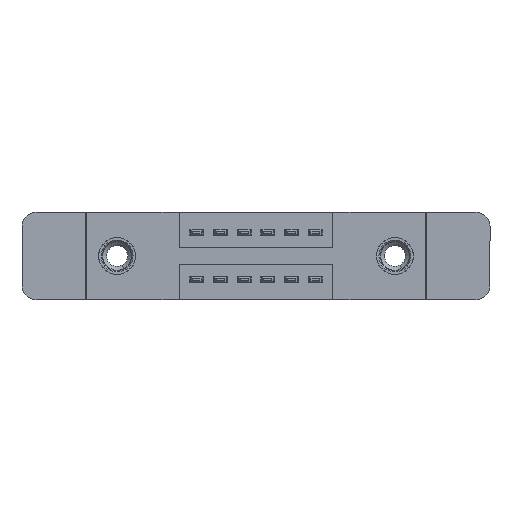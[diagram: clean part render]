
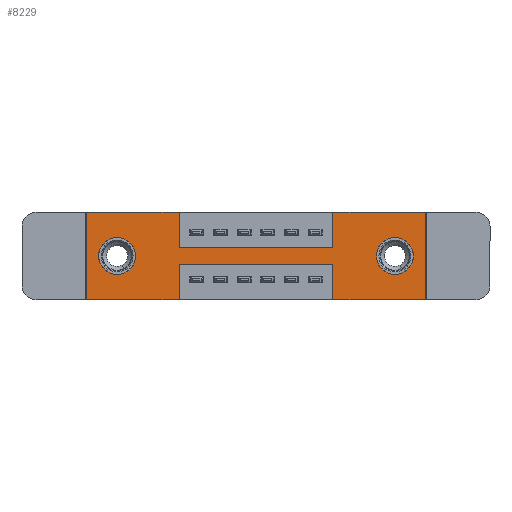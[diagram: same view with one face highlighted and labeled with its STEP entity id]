
A CAD part, front view. The second image highlights one B-rep face of the part: STEP entity #8229.
In plain terms, the highlighted planar face has unit normal (0, -1, 0).
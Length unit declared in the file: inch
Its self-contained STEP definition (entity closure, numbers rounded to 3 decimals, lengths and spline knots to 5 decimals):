
#13 = VERTEX_POINT ( 'NONE', #4931 ) ;
#34 = VECTOR ( 'NONE', #6083, 39.37008 ) ;
#103 = VERTEX_POINT ( 'NONE', #6002 ) ;
#179 = EDGE_CURVE ( 'NONE', #3154, #9858, #12522, .T. ) ;
#184 = EDGE_CURVE ( 'NONE', #6403, #9594, #1113, .T. ) ;
#365 = LINE ( 'NONE', #12591, #5651 ) ;
#390 = LINE ( 'NONE', #4262, #11974 ) ;
#586 = CARTESIAN_POINT ( 'NONE',  ( 0.3925, 0., 0. ) ) ;
#679 = CARTESIAN_POINT ( 'NONE',  ( 0., 0., 0. ) ) ;
#789 = CARTESIAN_POINT ( 'NONE',  ( 0.13, 0., -0.185 ) ) ;
#840 = DIRECTION ( 'NONE',  ( 0., 1., 0. ) ) ;
#951 = ORIENTED_EDGE ( 'NONE', *, *, #13408, .F. ) ;
#1021 = LINE ( 'NONE', #586, #12077 ) ;
#1113 = LINE ( 'NONE', #14376, #6379 ) ;
#1267 = CARTESIAN_POINT ( 'NONE',  ( 0.3925, 0., -0.15 ) ) ;
#1517 = EDGE_LOOP ( 'NONE', ( #12231, #14023 ) ) ;
#1647 = CARTESIAN_POINT ( 'NONE',  ( 1.435, 0., 0. ) ) ;
#1677 = DIRECTION ( 'NONE',  ( 0., 1., 0. ) ) ;
#1703 = CARTESIAN_POINT ( 'NONE',  ( 1.0425, 0., -0.37 ) ) ;
#1731 = CARTESIAN_POINT ( 'NONE',  ( 0.3925, 0., -0.15 ) ) ;
#1890 = DIRECTION ( 'NONE',  ( 0., 0., -1. ) ) ;
#1910 = DIRECTION ( 'NONE',  ( 0., 0., -1. ) ) ;
#2018 = ORIENTED_EDGE ( 'NONE', *, *, #8584, .F. ) ;
#2184 = LINE ( 'NONE', #1731, #4458 ) ;
#2248 = VERTEX_POINT ( 'NONE', #9121 ) ;
#2334 = CARTESIAN_POINT ( 'NONE',  ( 0., 0., -0.37 ) ) ;
#2453 = FACE_BOUND ( 'NONE', #1517, .T. ) ;
#2501 = EDGE_CURVE ( 'NONE', #13474, #6403, #12285, .T. ) ;
#2504 = VERTEX_POINT ( 'NONE', #7017 ) ;
#2559 = DIRECTION ( 'NONE',  ( 0., 0., -1. ) ) ;
#2589 = EDGE_CURVE ( 'NONE', #9858, #2504, #5633, .T. ) ;
#2788 = CARTESIAN_POINT ( 'NONE',  ( 0.3925, 0., -0.37 ) ) ;
#3071 = DIRECTION ( 'NONE',  ( 0., -1., 0. ) ) ;
#3099 = DIRECTION ( 'NONE',  ( 0., 0., 1. ) ) ;
#3154 = VERTEX_POINT ( 'NONE', #11383 ) ;
#3247 = EDGE_CURVE ( 'NONE', #10314, #103, #7860, .T. ) ;
#3334 = VECTOR ( 'NONE', #11514, 39.37008 ) ;
#3378 = ORIENTED_EDGE ( 'NONE', *, *, #11526, .F. ) ;
#3482 = CARTESIAN_POINT ( 'NONE',  ( 1.0425, 0., -0.37 ) ) ;
#3666 = FACE_OUTER_BOUND ( 'NONE', #9153, .T. ) ;
#3780 = VERTEX_POINT ( 'NONE', #1267 ) ;
#3973 = VECTOR ( 'NONE', #7808, 39.37008 ) ;
#4262 = CARTESIAN_POINT ( 'NONE',  ( 0., 0., -0.37 ) ) ;
#4344 = CARTESIAN_POINT ( 'NONE',  ( 1.0425, 0., 0. ) ) ;
#4386 = EDGE_CURVE ( 'NONE', #2504, #12737, #6975, .T. ) ;
#4458 = VECTOR ( 'NONE', #7306, 39.37008 ) ;
#4931 = CARTESIAN_POINT ( 'NONE',  ( 0.3925, 0., 0. ) ) ;
#4966 = CARTESIAN_POINT ( 'NONE',  ( 1.305, 0., -0.263 ) ) ;
#5084 = FACE_BOUND ( 'NONE', #12744, .T. ) ;
#5286 = PLANE ( 'NONE',  #10248 ) ;
#5414 = VECTOR ( 'NONE', #13587, 39.37008 ) ;
#5595 = CIRCLE ( 'NONE', #7825, 0.078 ) ;
#5633 = LINE ( 'NONE', #2788, #6839 ) ;
#5651 = VECTOR ( 'NONE', #8076, 39.37008 ) ;
#5856 = EDGE_CURVE ( 'NONE', #12737, #10537, #365, .T. ) ;
#5975 = ORIENTED_EDGE ( 'NONE', *, *, #12902, .F. ) ;
#6002 = CARTESIAN_POINT ( 'NONE',  ( 1.305, 0., -0.107 ) ) ;
#6014 = ORIENTED_EDGE ( 'NONE', *, *, #9058, .F. ) ;
#6083 = DIRECTION ( 'NONE',  ( 1., 0., 0. ) ) ;
#6117 = CARTESIAN_POINT ( 'NONE',  ( 0.13, 0., -0.263 ) ) ;
#6137 = CARTESIAN_POINT ( 'NONE',  ( 1.435, 0., 0. ) ) ;
#6379 = VECTOR ( 'NONE', #14284, 39.37008 ) ;
#6403 = VERTEX_POINT ( 'NONE', #4344 ) ;
#6425 = CARTESIAN_POINT ( 'NONE',  ( 0.13, 0., -0.185 ) ) ;
#6567 = DIRECTION ( 'NONE',  ( 0., 1., 0. ) ) ;
#6796 = DIRECTION ( 'NONE',  ( -1., 0., 0. ) ) ;
#6839 = VECTOR ( 'NONE', #9716, 39.37008 ) ;
#6975 = LINE ( 'NONE', #13548, #3973 ) ;
#7017 = CARTESIAN_POINT ( 'NONE',  ( 0.3925, 0., -0.37 ) ) ;
#7021 = ORIENTED_EDGE ( 'NONE', *, *, #3247, .T. ) ;
#7306 = DIRECTION ( 'NONE',  ( 1., 0., 0. ) ) ;
#7308 = CARTESIAN_POINT ( 'NONE',  ( 1.305, 0., -0.185 ) ) ;
#7399 = DIRECTION ( 'NONE',  ( 0., 1., 0. ) ) ;
#7406 = LINE ( 'NONE', #6137, #13202 ) ;
#7485 = CARTESIAN_POINT ( 'NONE',  ( 1.0425, 0., -0.15 ) ) ;
#7808 = DIRECTION ( 'NONE',  ( -1., 0., 0. ) ) ;
#7825 = AXIS2_PLACEMENT_3D ( 'NONE', #789, #840, #8484 ) ;
#7860 = CIRCLE ( 'NONE', #9550, 0.078 ) ;
#7888 = CARTESIAN_POINT ( 'NONE',  ( 0., 0., 0. ) ) ;
#7907 = VERTEX_POINT ( 'NONE', #1703 ) ;
#8076 = DIRECTION ( 'NONE',  ( 0., 0., 1. ) ) ;
#8165 = DIRECTION ( 'NONE',  ( -1., 0., 0. ) ) ;
#8229 = ADVANCED_FACE ( 'NONE', ( #5084, #2453, #3666 ), #5286, .T. ) ;
#8246 = CARTESIAN_POINT ( 'NONE',  ( 0.3925, 0., -0.22 ) ) ;
#8484 = DIRECTION ( 'NONE',  ( 0., 0., 1. ) ) ;
#8499 = CARTESIAN_POINT ( 'NONE',  ( 0., 0., -0.37 ) ) ;
#8504 = CARTESIAN_POINT ( 'NONE',  ( 0.3925, 0., -0.22 ) ) ;
#8584 = EDGE_CURVE ( 'NONE', #13, #3780, #1021, .T. ) ;
#8759 = EDGE_CURVE ( 'NONE', #9626, #2248, #5595, .T. ) ;
#8824 = LINE ( 'NONE', #7888, #34 ) ;
#8974 = ORIENTED_EDGE ( 'NONE', *, *, #13702, .F. ) ;
#9058 = EDGE_CURVE ( 'NONE', #7907, #3154, #13832, .T. ) ;
#9121 = CARTESIAN_POINT ( 'NONE',  ( 0.13, 0., -0.107 ) ) ;
#9153 = EDGE_LOOP ( 'NONE', ( #11688, #9285, #6014, #8974, #951, #13874, #13349, #5975, #2018, #3378, #14168, #13555 ) ) ;
#9216 = ORIENTED_EDGE ( 'NONE', *, *, #10294, .T. ) ;
#9285 = ORIENTED_EDGE ( 'NONE', *, *, #179, .F. ) ;
#9550 = AXIS2_PLACEMENT_3D ( 'NONE', #11020, #6567, #1910 ) ;
#9594 = VERTEX_POINT ( 'NONE', #1647 ) ;
#9626 = VERTEX_POINT ( 'NONE', #6117 ) ;
#9716 = DIRECTION ( 'NONE',  ( 0., 0., -1. ) ) ;
#9858 = VERTEX_POINT ( 'NONE', #8504 ) ;
#10248 = AXIS2_PLACEMENT_3D ( 'NONE', #8499, #3071, #1890 ) ;
#10294 = EDGE_CURVE ( 'NONE', #103, #10314, #11318, .T. ) ;
#10314 = VERTEX_POINT ( 'NONE', #4966 ) ;
#10537 = VERTEX_POINT ( 'NONE', #679 ) ;
#11020 = CARTESIAN_POINT ( 'NONE',  ( 1.305, 0., -0.185 ) ) ;
#11065 = CARTESIAN_POINT ( 'NONE',  ( 1.435, 0., -0.37 ) ) ;
#11318 = CIRCLE ( 'NONE', #13856, 0.078 ) ;
#11383 = CARTESIAN_POINT ( 'NONE',  ( 1.0425, 0., -0.22 ) ) ;
#11514 = DIRECTION ( 'NONE',  ( 0., 0., 1. ) ) ;
#11526 = EDGE_CURVE ( 'NONE', #10537, #13, #8824, .T. ) ;
#11613 = CARTESIAN_POINT ( 'NONE',  ( 1.0425, 0., 0. ) ) ;
#11688 = ORIENTED_EDGE ( 'NONE', *, *, #2589, .F. ) ;
#11893 = VERTEX_POINT ( 'NONE', #11065 ) ;
#11974 = VECTOR ( 'NONE', #6796, 39.37008 ) ;
#12077 = VECTOR ( 'NONE', #14004, 39.37008 ) ;
#12231 = ORIENTED_EDGE ( 'NONE', *, *, #12989, .T. ) ;
#12285 = LINE ( 'NONE', #11613, #3334 ) ;
#12522 = LINE ( 'NONE', #8246, #13757 ) ;
#12591 = CARTESIAN_POINT ( 'NONE',  ( 0., 0., 0. ) ) ;
#12737 = VERTEX_POINT ( 'NONE', #2334 ) ;
#12744 = EDGE_LOOP ( 'NONE', ( #9216, #7021 ) ) ;
#12902 = EDGE_CURVE ( 'NONE', #3780, #13474, #2184, .T. ) ;
#12989 = EDGE_CURVE ( 'NONE', #2248, #9626, #14285, .T. ) ;
#13202 = VECTOR ( 'NONE', #2559, 39.37008 ) ;
#13230 = AXIS2_PLACEMENT_3D ( 'NONE', #6425, #7399, #3099 ) ;
#13349 = ORIENTED_EDGE ( 'NONE', *, *, #2501, .F. ) ;
#13408 = EDGE_CURVE ( 'NONE', #9594, #11893, #7406, .T. ) ;
#13474 = VERTEX_POINT ( 'NONE', #7485 ) ;
#13548 = CARTESIAN_POINT ( 'NONE',  ( 0., 0., -0.37 ) ) ;
#13555 = ORIENTED_EDGE ( 'NONE', *, *, #4386, .F. ) ;
#13587 = DIRECTION ( 'NONE',  ( 0., 0., 1. ) ) ;
#13702 = EDGE_CURVE ( 'NONE', #11893, #7907, #390, .T. ) ;
#13757 = VECTOR ( 'NONE', #8165, 39.37008 ) ;
#13832 = LINE ( 'NONE', #3482, #5414 ) ;
#13856 = AXIS2_PLACEMENT_3D ( 'NONE', #7308, #1677, #13949 ) ;
#13874 = ORIENTED_EDGE ( 'NONE', *, *, #184, .F. ) ;
#13949 = DIRECTION ( 'NONE',  ( 0., 0., -1. ) ) ;
#14004 = DIRECTION ( 'NONE',  ( 0., 0., -1. ) ) ;
#14023 = ORIENTED_EDGE ( 'NONE', *, *, #8759, .T. ) ;
#14168 = ORIENTED_EDGE ( 'NONE', *, *, #5856, .F. ) ;
#14284 = DIRECTION ( 'NONE',  ( 1., 0., 0. ) ) ;
#14285 = CIRCLE ( 'NONE', #13230, 0.078 ) ;
#14376 = CARTESIAN_POINT ( 'NONE',  ( 0., 0., 0. ) ) ;
